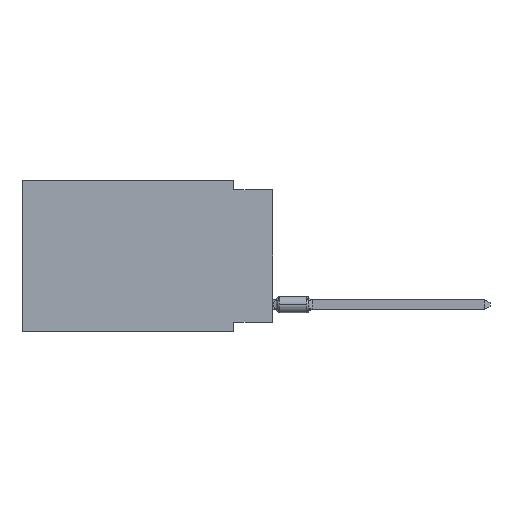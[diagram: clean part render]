
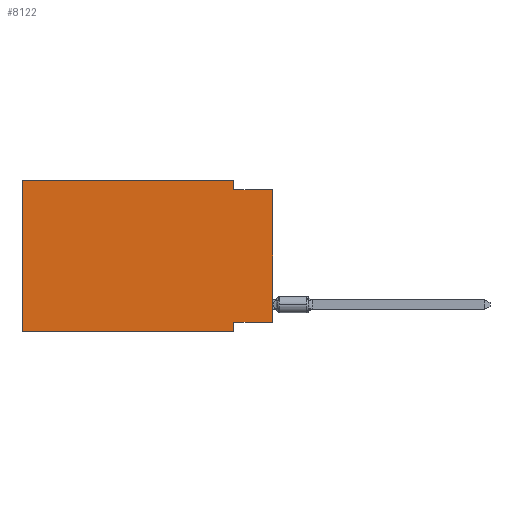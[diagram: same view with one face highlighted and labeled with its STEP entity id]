
A CAD part, left-side view. The second image highlights one B-rep face of the part: STEP entity #8122.
In plain terms, the highlighted planar face has unit normal (-1, 0, 0).
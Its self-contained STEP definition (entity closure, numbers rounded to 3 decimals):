
#251 = ORIENTED_EDGE ( 'NONE', *, *, #9894, .F. ) ;
#267 = EDGE_CURVE ( 'NONE', #8013, #4305, #6737, .T. ) ;
#308 = EDGE_CURVE ( 'NONE', #17786, #15215, #2577, .T. ) ;
#1450 = VERTEX_POINT ( 'NONE', #10659 ) ;
#1671 = CARTESIAN_POINT ( 'NONE',  ( 0., 16.383, 0. ) ) ;
#2577 = LINE ( 'NONE', #15239, #5110 ) ;
#2612 = DIRECTION ( 'NONE',  ( 0., 0., 1. ) ) ;
#2675 = CARTESIAN_POINT ( 'NONE',  ( 0., 2.54, 0. ) ) ;
#2749 = CARTESIAN_POINT ( 'NONE',  ( 0., 2.54, -9.906 ) ) ;
#3051 = DIRECTION ( 'NONE',  ( 0., -1., 0. ) ) ;
#3093 = DIRECTION ( 'NONE',  ( 0., 1., 0. ) ) ;
#3119 = PLANE ( 'NONE',  #14385 ) ;
#3896 = CARTESIAN_POINT ( 'NONE',  ( 0., 16.383, 0. ) ) ;
#3999 = CARTESIAN_POINT ( 'NONE',  ( 0., 16.383, 0. ) ) ;
#4157 = LINE ( 'NONE', #1671, #14338 ) ;
#4305 = VERTEX_POINT ( 'NONE', #10701 ) ;
#4535 = CARTESIAN_POINT ( 'NONE',  ( 0., 2.54, 0. ) ) ;
#4822 = DIRECTION ( 'NONE',  ( 0., 0., -1. ) ) ;
#5014 = EDGE_CURVE ( 'NONE', #8259, #8013, #12791, .T. ) ;
#5059 = VECTOR ( 'NONE', #7755, 1000. ) ;
#5110 = VECTOR ( 'NONE', #16205, 1000. ) ;
#5264 = DIRECTION ( 'NONE',  ( 0., 0., -1. ) ) ;
#5506 = VERTEX_POINT ( 'NONE', #2675 ) ;
#6737 = LINE ( 'NONE', #2749, #9811 ) ;
#7273 = DIRECTION ( 'NONE',  ( 0., 0., -1. ) ) ;
#7571 = CARTESIAN_POINT ( 'NONE',  ( 0., 0., 0. ) ) ;
#7755 = DIRECTION ( 'NONE',  ( 0., 0., 1. ) ) ;
#8013 = VERTEX_POINT ( 'NONE', #11332 ) ;
#8122 = ADVANCED_FACE ( 'NONE', ( #11520 ), #3119, .F. ) ;
#8259 = VERTEX_POINT ( 'NONE', #12075 ) ;
#8603 = CARTESIAN_POINT ( 'NONE',  ( 0., 16.383, -9.906 ) ) ;
#8940 = CARTESIAN_POINT ( 'NONE',  ( 0., 16.383, 0. ) ) ;
#9811 = VECTOR ( 'NONE', #5264, 1000. ) ;
#9894 = EDGE_CURVE ( 'NONE', #5506, #17786, #17189, .T. ) ;
#10030 = ORIENTED_EDGE ( 'NONE', *, *, #5014, .F. ) ;
#10659 = CARTESIAN_POINT ( 'NONE',  ( 0., 16.383, -9.906 ) ) ;
#10701 = CARTESIAN_POINT ( 'NONE',  ( 0., 2.54, -9.906 ) ) ;
#11094 = DIRECTION ( 'NONE',  ( 0., -1., 0. ) ) ;
#11332 = CARTESIAN_POINT ( 'NONE',  ( 0., 2.54, -9.271 ) ) ;
#11480 = VECTOR ( 'NONE', #4822, 1000. ) ;
#11520 = FACE_OUTER_BOUND ( 'NONE', #17974, .T. ) ;
#12075 = CARTESIAN_POINT ( 'NONE',  ( 0., 0., -9.271 ) ) ;
#12791 = LINE ( 'NONE', #15744, #16171 ) ;
#12793 = ORIENTED_EDGE ( 'NONE', *, *, #12892, .T. ) ;
#12889 = ORIENTED_EDGE ( 'NONE', *, *, #308, .F. ) ;
#12892 = EDGE_CURVE ( 'NONE', #1450, #4305, #15348, .T. ) ;
#13490 = ORIENTED_EDGE ( 'NONE', *, *, #15618, .T. ) ;
#13947 = CARTESIAN_POINT ( 'NONE',  ( 0., 2.54, -0.635 ) ) ;
#14338 = VECTOR ( 'NONE', #3051, 1000. ) ;
#14385 = AXIS2_PLACEMENT_3D ( 'NONE', #8940, #15585, #7273 ) ;
#14410 = VERTEX_POINT ( 'NONE', #3896 ) ;
#14718 = ORIENTED_EDGE ( 'NONE', *, *, #17119, .F. ) ;
#15215 = VERTEX_POINT ( 'NONE', #16379 ) ;
#15239 = CARTESIAN_POINT ( 'NONE',  ( 0., 0., -0.635 ) ) ;
#15348 = LINE ( 'NONE', #8603, #17553 ) ;
#15585 = DIRECTION ( 'NONE',  ( 1., 0., 0. ) ) ;
#15618 = EDGE_CURVE ( 'NONE', #8259, #15215, #15968, .T. ) ;
#15744 = CARTESIAN_POINT ( 'NONE',  ( 0., 0., -9.271 ) ) ;
#15968 = LINE ( 'NONE', #7571, #5059 ) ;
#16171 = VECTOR ( 'NONE', #3093, 1000. ) ;
#16205 = DIRECTION ( 'NONE',  ( 0., -1., 0. ) ) ;
#16379 = CARTESIAN_POINT ( 'NONE',  ( 0., 0., -0.635 ) ) ;
#16865 = ORIENTED_EDGE ( 'NONE', *, *, #267, .F. ) ;
#16901 = VECTOR ( 'NONE', #2612, 1000. ) ;
#17053 = ORIENTED_EDGE ( 'NONE', *, *, #17764, .F. ) ;
#17119 = EDGE_CURVE ( 'NONE', #1450, #14410, #18045, .T. ) ;
#17189 = LINE ( 'NONE', #4535, #11480 ) ;
#17553 = VECTOR ( 'NONE', #11094, 1000. ) ;
#17764 = EDGE_CURVE ( 'NONE', #14410, #5506, #4157, .T. ) ;
#17786 = VERTEX_POINT ( 'NONE', #13947 ) ;
#17974 = EDGE_LOOP ( 'NONE', ( #13490, #12889, #251, #17053, #14718, #12793, #16865, #10030 ) ) ;
#18045 = LINE ( 'NONE', #3999, #16901 ) ;
